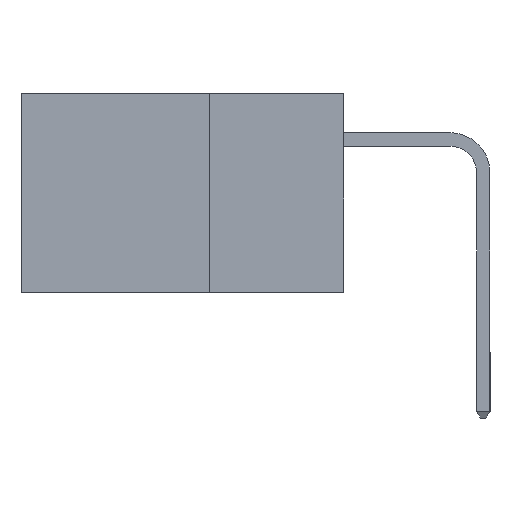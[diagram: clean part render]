
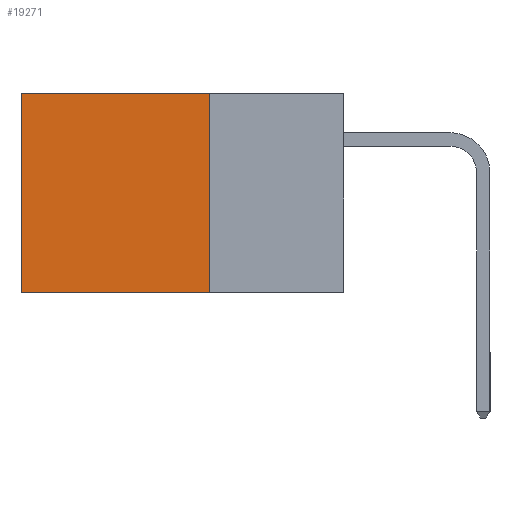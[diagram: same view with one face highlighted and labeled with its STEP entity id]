
A CAD part, left-side view. The second image highlights one B-rep face of the part: STEP entity #19271.
In plain terms, the highlighted planar face has unit normal (-1, 0, 0).
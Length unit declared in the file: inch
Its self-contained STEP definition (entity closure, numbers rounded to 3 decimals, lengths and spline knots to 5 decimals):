
#67 = VERTEX_POINT ( 'NONE', #7271 ) ;
#510 = VECTOR ( 'NONE', #9964, 39.37008 ) ;
#970 = VERTEX_POINT ( 'NONE', #20384 ) ;
#1247 = LINE ( 'NONE', #2778, #2186 ) ;
#2018 = CARTESIAN_POINT ( 'NONE',  ( 0.2615, 0.25, 0. ) ) ;
#2186 = VECTOR ( 'NONE', #11439, 39.37008 ) ;
#2778 = CARTESIAN_POINT ( 'NONE',  ( 0.2615, 0.25, -0.37 ) ) ;
#4228 = DIRECTION ( 'NONE',  ( 0., 1., 0. ) ) ;
#4683 = EDGE_CURVE ( 'NONE', #18615, #970, #7307, .T. ) ;
#4785 = FACE_OUTER_BOUND ( 'NONE', #14890, .T. ) ;
#5335 = VECTOR ( 'NONE', #4228, 39.37008 ) ;
#6267 = ORIENTED_EDGE ( 'NONE', *, *, #8341, .F. ) ;
#6531 = DIRECTION ( 'NONE',  ( 0., 0., -1. ) ) ;
#7271 = CARTESIAN_POINT ( 'NONE',  ( 0.2615, 0.6, -0.37 ) ) ;
#7288 = CARTESIAN_POINT ( 'NONE',  ( 0.2615, 0.25, -0.37 ) ) ;
#7307 = LINE ( 'NONE', #15549, #5335 ) ;
#7717 = CARTESIAN_POINT ( 'NONE',  ( 0.2615, 0.6, -0.37 ) ) ;
#7826 = DIRECTION ( 'NONE',  ( 0., 0., -1. ) ) ;
#7968 = DIRECTION ( 'NONE',  ( 1., 0., 0. ) ) ;
#8077 = CARTESIAN_POINT ( 'NONE',  ( 0.2615, 0.25, -0.37 ) ) ;
#8341 = EDGE_CURVE ( 'NONE', #18615, #21085, #8818, .T. ) ;
#8818 = LINE ( 'NONE', #11611, #510 ) ;
#9964 = DIRECTION ( 'NONE',  ( 0., 0., -1. ) ) ;
#10476 = ORIENTED_EDGE ( 'NONE', *, *, #21157, .T. ) ;
#11439 = DIRECTION ( 'NONE',  ( 0., 1., 0. ) ) ;
#11611 = CARTESIAN_POINT ( 'NONE',  ( 0.2615, 0.25, -0.37 ) ) ;
#12206 = AXIS2_PLACEMENT_3D ( 'NONE', #8077, #7968, #6531 ) ;
#12470 = EDGE_CURVE ( 'NONE', #21085, #67, #1247, .T. ) ;
#12600 = VECTOR ( 'NONE', #7826, 39.37008 ) ;
#14890 = EDGE_LOOP ( 'NONE', ( #10476, #19149, #6267, #20797 ) ) ;
#15549 = CARTESIAN_POINT ( 'NONE',  ( 0.2615, 0.25, 0. ) ) ;
#18615 = VERTEX_POINT ( 'NONE', #2018 ) ;
#19149 = ORIENTED_EDGE ( 'NONE', *, *, #12470, .F. ) ;
#19271 = ADVANCED_FACE ( 'NONE', ( #4785 ), #19912, .F. ) ;
#19769 = LINE ( 'NONE', #7717, #12600 ) ;
#19912 = PLANE ( 'NONE',  #12206 ) ;
#20384 = CARTESIAN_POINT ( 'NONE',  ( 0.2615, 0.6, 0. ) ) ;
#20797 = ORIENTED_EDGE ( 'NONE', *, *, #4683, .T. ) ;
#21085 = VERTEX_POINT ( 'NONE', #7288 ) ;
#21157 = EDGE_CURVE ( 'NONE', #970, #67, #19769, .T. ) ;
